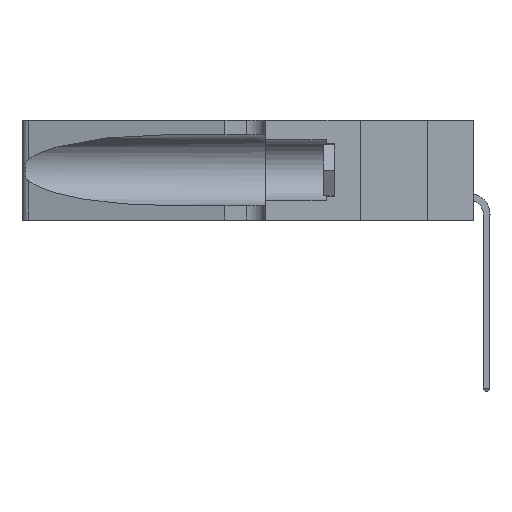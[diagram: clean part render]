
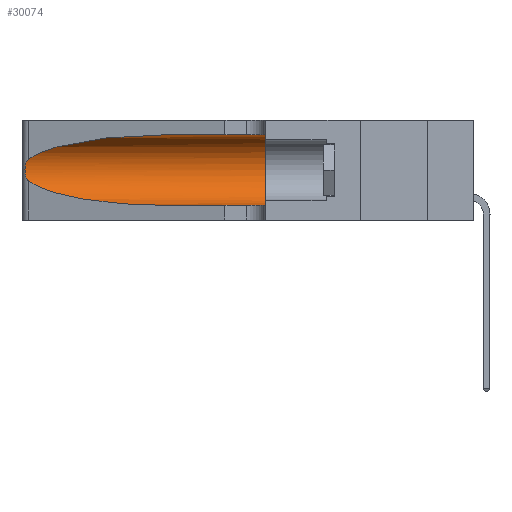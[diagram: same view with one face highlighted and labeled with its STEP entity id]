
A CAD part, left-side view. The second image highlights one B-rep face of the part: STEP entity #30074.
In plain terms, the highlighted cylindrical face has radius 3.308 mm (diameter 6.617 mm), a partial arc.
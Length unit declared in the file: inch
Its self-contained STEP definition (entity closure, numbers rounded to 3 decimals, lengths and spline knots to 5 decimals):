
#485 = CARTESIAN_POINT ( 'NONE',  ( 0.18966, 0.96281, 0.05475 ) ) ;
#988 = FACE_OUTER_BOUND ( 'NONE', #5599, .T. ) ;
#1034 = VERTEX_POINT ( 'NONE', #36979 ) ;
#3333 = DIRECTION ( 'NONE',  ( 0., 0., -1. ) ) ;
#3671 = CARTESIAN_POINT ( 'NONE',  ( 0.1305, 0.35, 0.185 ) ) ;
#4103 = CIRCLE ( 'NONE', #35731, 0.13025 ) ;
#5599 = EDGE_LOOP ( 'NONE', ( #5687, #32975, #22755, #35925, #26066, #17568 ) ) ;
#5687 = ORIENTED_EDGE ( 'NONE', *, *, #8941, .T. ) ;
#6458 = CARTESIAN_POINT ( 'NONE',  ( 0.25787, 1.23484, 0.2124 ) ) ;
#6518 = CARTESIAN_POINT ( 'NONE',  ( 0.1305, 1.61858, 0.185 ) ) ;
#6599 = CARTESIAN_POINT ( 'NONE',  ( 0.25789, 1.23486, 0.15765 ) ) ;
#6958 = EDGE_CURVE ( 'NONE', #25913, #32862, #28845, .T. ) ;
#8301 = CARTESIAN_POINT ( 'NONE',  ( 0.18966, 0.96281, 0.31525 ) ) ;
#8838 = EDGE_CURVE ( 'NONE', #8882, #1034, #19109, .T. ) ;
#8882 = VERTEX_POINT ( 'NONE', #24462 ) ;
#8941 = EDGE_CURVE ( 'NONE', #25913, #9974, #23947, .T. ) ;
#9421 = CARTESIAN_POINT ( 'NONE',  ( 0.25856, 1.23593, 0.16098 ) ) ;
#9974 = VERTEX_POINT ( 'NONE', #36853 ) ;
#10599 = VECTOR ( 'NONE', #19390, 39.37008 ) ;
#12237 = DIRECTION ( 'NONE',  ( 0., 0., 1. ) ) ;
#12478 = CARTESIAN_POINT ( 'NONE',  ( 0.26017, 1.23833, 0.17102 ) ) ;
#12620 = DIRECTION ( 'NONE',  ( 0., -1., 0. ) ) ;
#15182 = CARTESIAN_POINT ( 'NONE',  ( 0.26075, 1.23896, 0.19203 ) ) ;
#15444 = CARTESIAN_POINT ( 'NONE',  ( 0.25555, 1.22993, 0.14849 ) ) ;
#15580 = CARTESIAN_POINT ( 'NONE',  ( 0.25639, 1.23184, 0.21858 ) ) ;
#15730 = CARTESIAN_POINT ( 'NONE',  ( 0.1305, 1.61858, 0.05475 ) ) ;
#17568 = ORIENTED_EDGE ( 'NONE', *, *, #6958, .F. ) ;
#17933 = EDGE_CURVE ( 'NONE', #32862, #1034, #4103, .T. ) ;
#17995 = CARTESIAN_POINT ( 'NONE',  ( 0.2373, 1.15595, 0.08982 ) ) ;
#18079 = CARTESIAN_POINT ( 'NONE',  ( 0.26075, 1.23896, 0.178 ) ) ;
#18080 = EDGE_CURVE ( 'NONE', #9974, #23630, #18858, .T. ) ;
#18269 = DIRECTION ( 'NONE',  ( 0., -1., 0. ) ) ;
#18738 = CARTESIAN_POINT ( 'NONE',  ( 0.1305, 0.35, 0.31525 ) ) ;
#18858 = B_SPLINE_CURVE_WITH_KNOTS ( 'NONE', 3,
 ( #23788, #27137, #15580, #6458, #26743, #29653, #15182, #18079, #12478, #9421, #6599, #21255, #15444, #35855 ),
 .UNSPECIFIED., .F., .F.,
 ( 4, 2, 2, 2, 2, 2, 4 ),
 ( 0., 0.00027, 0.00053, 0.00107, 0.0016, 0.00187, 0.00214 ),
 .UNSPECIFIED. ) ;
#19109 = LINE ( 'NONE', #15730, #29542 ) ;
#19390 = DIRECTION ( 'NONE',  ( 0., -1., 0. ) ) ;
#21255 = CARTESIAN_POINT ( 'NONE',  ( 0.25639, 1.23186, 0.15144 ) ) ;
#22318 = EDGE_CURVE ( 'NONE', #23630, #8882, #28005, .T. ) ;
#22755 = ORIENTED_EDGE ( 'NONE', *, *, #22318, .T. ) ;
#22927 = CYLINDRICAL_SURFACE ( 'NONE', #23684, 0.13025 ) ;
#23154 = CARTESIAN_POINT ( 'NONE',  ( 0.25487, 1.22718, 0.22369 ) ) ;
#23630 = VERTEX_POINT ( 'NONE', #31166 ) ;
#23684 = AXIS2_PLACEMENT_3D ( 'NONE', #6518, #18269, #3333 ) ;
#23788 = CARTESIAN_POINT ( 'NONE',  ( 0.25487, 1.22718, 0.22369 ) ) ;
#23822 = CARTESIAN_POINT ( 'NONE',  ( 0.1305, 0.72297, 0.05475 ) ) ;
#23947 =( BOUNDED_CURVE ( )  B_SPLINE_CURVE ( 3, ( #28557, #8301, #37501, #23154 ),
 .UNSPECIFIED., .F., .T. ) 
 B_SPLINE_CURVE_WITH_KNOTS ( ( 4, 4 ),
 ( 1.5708, 2.84003 ),
 .UNSPECIFIED. ) 
 CURVE ( )  GEOMETRIC_REPRESENTATION_ITEM ( )  RATIONAL_B_SPLINE_CURVE ( ( 1., 0.87, 0.87, 1. ) ) 
 REPRESENTATION_ITEM ( '' )  );
#24462 = CARTESIAN_POINT ( 'NONE',  ( 0.1305, 0.72297, 0.05475 ) ) ;
#25913 = VERTEX_POINT ( 'NONE', #30213 ) ;
#26066 = ORIENTED_EDGE ( 'NONE', *, *, #17933, .F. ) ;
#26743 = CARTESIAN_POINT ( 'NONE',  ( 0.25854, 1.2359, 0.20912 ) ) ;
#27137 = CARTESIAN_POINT ( 'NONE',  ( 0.25555, 1.22994, 0.2215 ) ) ;
#28005 =( BOUNDED_CURVE ( )  B_SPLINE_CURVE ( 3, ( #35390, #17995, #485, #23822 ),
 .UNSPECIFIED., .F., .F. ) 
 B_SPLINE_CURVE_WITH_KNOTS ( ( 4, 4 ),
 ( 3.44316, 4.71239 ),
 .UNSPECIFIED. ) 
 CURVE ( )  GEOMETRIC_REPRESENTATION_ITEM ( )  RATIONAL_B_SPLINE_CURVE ( ( 1., 0.87, 0.87, 1. ) ) 
 REPRESENTATION_ITEM ( '' )  );
#28557 = CARTESIAN_POINT ( 'NONE',  ( 0.1305, 0.72297, 0.31525 ) ) ;
#28845 = LINE ( 'NONE', #30702, #10599 ) ;
#29542 = VECTOR ( 'NONE', #12620, 39.37008 ) ;
#29653 = CARTESIAN_POINT ( 'NONE',  ( 0.26018, 1.23835, 0.19895 ) ) ;
#30074 = ADVANCED_FACE ( 'NONE', ( #988 ), #22927, .F. ) ;
#30213 = CARTESIAN_POINT ( 'NONE',  ( 0.1305, 0.72297, 0.31525 ) ) ;
#30702 = CARTESIAN_POINT ( 'NONE',  ( 0.1305, 1.61858, 0.31525 ) ) ;
#31166 = CARTESIAN_POINT ( 'NONE',  ( 0.25487, 1.22718, 0.14631 ) ) ;
#32862 = VERTEX_POINT ( 'NONE', #18738 ) ;
#32975 = ORIENTED_EDGE ( 'NONE', *, *, #18080, .T. ) ;
#35390 = CARTESIAN_POINT ( 'NONE',  ( 0.25487, 1.22718, 0.14631 ) ) ;
#35731 = AXIS2_PLACEMENT_3D ( 'NONE', #3671, #35875, #12237 ) ;
#35855 = CARTESIAN_POINT ( 'NONE',  ( 0.25487, 1.22718, 0.14631 ) ) ;
#35875 = DIRECTION ( 'NONE',  ( 0., 1., 0. ) ) ;
#35925 = ORIENTED_EDGE ( 'NONE', *, *, #8838, .T. ) ;
#36853 = CARTESIAN_POINT ( 'NONE',  ( 0.25487, 1.22718, 0.22369 ) ) ;
#36979 = CARTESIAN_POINT ( 'NONE',  ( 0.1305, 0.35, 0.05475 ) ) ;
#37501 = CARTESIAN_POINT ( 'NONE',  ( 0.2373, 1.15595, 0.28018 ) ) ;
